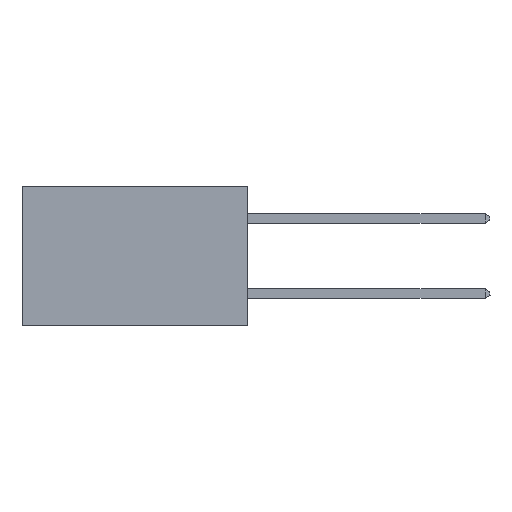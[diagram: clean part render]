
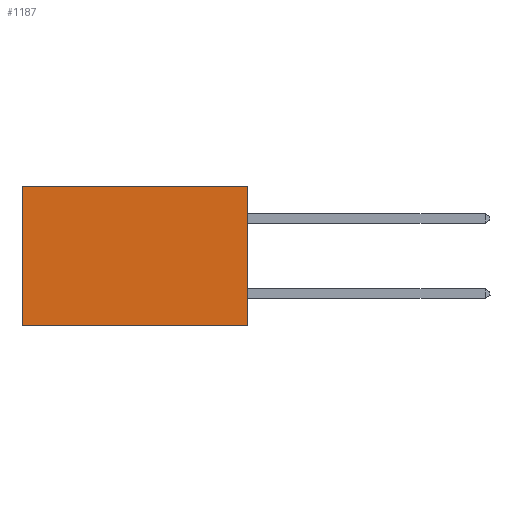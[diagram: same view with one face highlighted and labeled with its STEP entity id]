
A CAD part, left-side view. The second image highlights one B-rep face of the part: STEP entity #1187.
In plain terms, the highlighted planar face has unit normal (-1, 0, 0).
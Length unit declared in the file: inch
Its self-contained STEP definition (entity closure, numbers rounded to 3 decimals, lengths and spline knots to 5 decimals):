
#631 = VERTEX_POINT ( 'NONE', #1331 ) ;
#864 = EDGE_LOOP ( 'NONE', ( #8352, #5598, #19665, #17485 ) ) ;
#1187 = ADVANCED_FACE ( 'NONE', ( #5167 ), #6654, .F. ) ;
#1331 = CARTESIAN_POINT ( 'NONE',  ( 0.298, 0., 0. ) ) ;
#1859 = DIRECTION ( 'NONE',  ( 0., 1., 0. ) ) ;
#2017 = CARTESIAN_POINT ( 'NONE',  ( 0.298, 0., 0. ) ) ;
#2088 = DIRECTION ( 'NONE',  ( 0., 0., -1. ) ) ;
#2560 = CARTESIAN_POINT ( 'NONE',  ( 0.298, 0., 0. ) ) ;
#2842 = CARTESIAN_POINT ( 'NONE',  ( 0.298, 0.6, 0. ) ) ;
#4319 = EDGE_CURVE ( 'NONE', #631, #9366, #20894, .T. ) ;
#5103 = CARTESIAN_POINT ( 'NONE',  ( 0.298, 0., -0.37 ) ) ;
#5167 = FACE_OUTER_BOUND ( 'NONE', #864, .T. ) ;
#5283 = VECTOR ( 'NONE', #1859, 39.37008 ) ;
#5598 = ORIENTED_EDGE ( 'NONE', *, *, #7572, .F. ) ;
#6432 = VECTOR ( 'NONE', #13890, 39.37008 ) ;
#6438 = CARTESIAN_POINT ( 'NONE',  ( 0.298, 0., -0.37 ) ) ;
#6577 = DIRECTION ( 'NONE',  ( 0., 0., -1. ) ) ;
#6654 = PLANE ( 'NONE',  #12598 ) ;
#7040 = EDGE_CURVE ( 'NONE', #9399, #20275, #15345, .T. ) ;
#7572 = EDGE_CURVE ( 'NONE', #9366, #20275, #9690, .T. ) ;
#8352 = ORIENTED_EDGE ( 'NONE', *, *, #7040, .T. ) ;
#9366 = VERTEX_POINT ( 'NONE', #6438 ) ;
#9399 = VERTEX_POINT ( 'NONE', #2842 ) ;
#9690 = LINE ( 'NONE', #5103, #5283 ) ;
#10110 = DIRECTION ( 'NONE',  ( 0., 0., -1. ) ) ;
#11619 = VECTOR ( 'NONE', #2088, 39.37008 ) ;
#12131 = LINE ( 'NONE', #2560, #6432 ) ;
#12598 = AXIS2_PLACEMENT_3D ( 'NONE', #16475, #17998, #10110 ) ;
#13419 = CARTESIAN_POINT ( 'NONE',  ( 0.298, 0.6, 0. ) ) ;
#13890 = DIRECTION ( 'NONE',  ( 0., 1., 0. ) ) ;
#15088 = VECTOR ( 'NONE', #6577, 39.37008 ) ;
#15345 = LINE ( 'NONE', #13419, #15088 ) ;
#15918 = EDGE_CURVE ( 'NONE', #631, #9399, #12131, .T. ) ;
#16475 = CARTESIAN_POINT ( 'NONE',  ( 0.298, 0., 0. ) ) ;
#17444 = CARTESIAN_POINT ( 'NONE',  ( 0.298, 0.6, -0.37 ) ) ;
#17485 = ORIENTED_EDGE ( 'NONE', *, *, #15918, .T. ) ;
#17998 = DIRECTION ( 'NONE',  ( 1., 0., 0. ) ) ;
#19665 = ORIENTED_EDGE ( 'NONE', *, *, #4319, .F. ) ;
#20275 = VERTEX_POINT ( 'NONE', #17444 ) ;
#20894 = LINE ( 'NONE', #2017, #11619 ) ;
